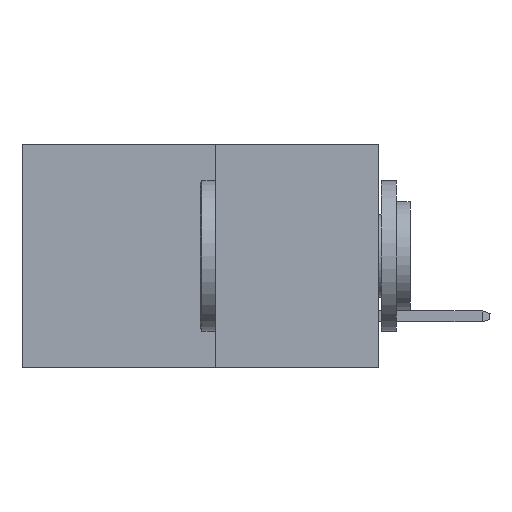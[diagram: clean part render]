
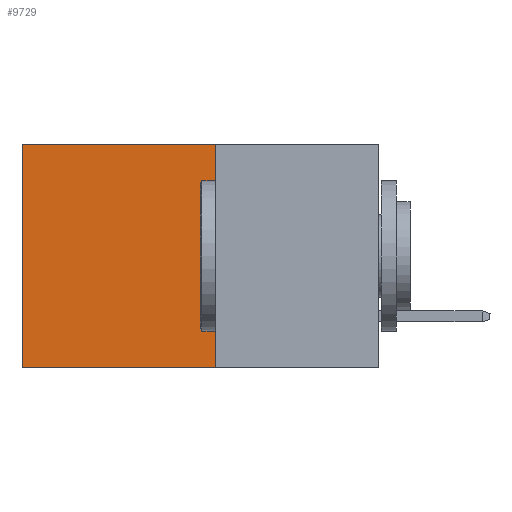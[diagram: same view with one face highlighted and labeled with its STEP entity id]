
A CAD part, left-side view. The second image highlights one B-rep face of the part: STEP entity #9729.
In plain terms, the highlighted planar face has unit normal (-1, 0, 0).
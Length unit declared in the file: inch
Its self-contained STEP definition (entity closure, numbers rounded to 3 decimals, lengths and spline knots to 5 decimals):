
#627 = VECTOR ( 'NONE', #4538, 39.37008 ) ;
#1264 = EDGE_LOOP ( 'NONE', ( #1609, #9672, #3430, #3747 ) ) ;
#1609 = ORIENTED_EDGE ( 'NONE', *, *, #4028, .T. ) ;
#1662 = CARTESIAN_POINT ( 'NONE',  ( 0.277, 0.27, -0.37 ) ) ;
#2081 = EDGE_CURVE ( 'NONE', #4301, #4638, #4365, .T. ) ;
#2309 = CARTESIAN_POINT ( 'NONE',  ( 0.277, 0.27, -0.37 ) ) ;
#2827 = AXIS2_PLACEMENT_3D ( 'NONE', #2309, #9140, #4780 ) ;
#2859 = LINE ( 'NONE', #3994, #627 ) ;
#3053 = VECTOR ( 'NONE', #4084, 39.37008 ) ;
#3086 = EDGE_CURVE ( 'NONE', #3775, #3282, #3318, .T. ) ;
#3282 = VERTEX_POINT ( 'NONE', #6349 ) ;
#3318 = LINE ( 'NONE', #5894, #3053 ) ;
#3430 = ORIENTED_EDGE ( 'NONE', *, *, #4787, .F. ) ;
#3747 = ORIENTED_EDGE ( 'NONE', *, *, #3086, .T. ) ;
#3775 = VERTEX_POINT ( 'NONE', #9856 ) ;
#3976 = PLANE ( 'NONE',  #2827 ) ;
#3994 = CARTESIAN_POINT ( 'NONE',  ( 0.277, 0.27, -0.37 ) ) ;
#4028 = EDGE_CURVE ( 'NONE', #3282, #4638, #6269, .T. ) ;
#4084 = DIRECTION ( 'NONE',  ( 0., 1., 0. ) ) ;
#4301 = VERTEX_POINT ( 'NONE', #8910 ) ;
#4365 = LINE ( 'NONE', #1662, #8107 ) ;
#4538 = DIRECTION ( 'NONE',  ( 0., 0., -1. ) ) ;
#4638 = VERTEX_POINT ( 'NONE', #4823 ) ;
#4780 = DIRECTION ( 'NONE',  ( 0., 0., -1. ) ) ;
#4787 = EDGE_CURVE ( 'NONE', #3775, #4301, #2859, .T. ) ;
#4823 = CARTESIAN_POINT ( 'NONE',  ( 0.277, 0.59, -0.37 ) ) ;
#5894 = CARTESIAN_POINT ( 'NONE',  ( 0.277, 0.27, 0. ) ) ;
#6269 = LINE ( 'NONE', #8720, #9574 ) ;
#6349 = CARTESIAN_POINT ( 'NONE',  ( 0.277, 0.59, 0. ) ) ;
#8107 = VECTOR ( 'NONE', #9761, 39.37008 ) ;
#8507 = FACE_OUTER_BOUND ( 'NONE', #1264, .T. ) ;
#8607 = DIRECTION ( 'NONE',  ( 0., 0., -1. ) ) ;
#8720 = CARTESIAN_POINT ( 'NONE',  ( 0.277, 0.59, -0.37 ) ) ;
#8910 = CARTESIAN_POINT ( 'NONE',  ( 0.277, 0.27, -0.37 ) ) ;
#9140 = DIRECTION ( 'NONE',  ( 1., 0., 0. ) ) ;
#9574 = VECTOR ( 'NONE', #8607, 39.37008 ) ;
#9672 = ORIENTED_EDGE ( 'NONE', *, *, #2081, .F. ) ;
#9729 = ADVANCED_FACE ( 'NONE', ( #8507 ), #3976, .F. ) ;
#9761 = DIRECTION ( 'NONE',  ( 0., 1., 0. ) ) ;
#9856 = CARTESIAN_POINT ( 'NONE',  ( 0.277, 0.27, 0. ) ) ;
